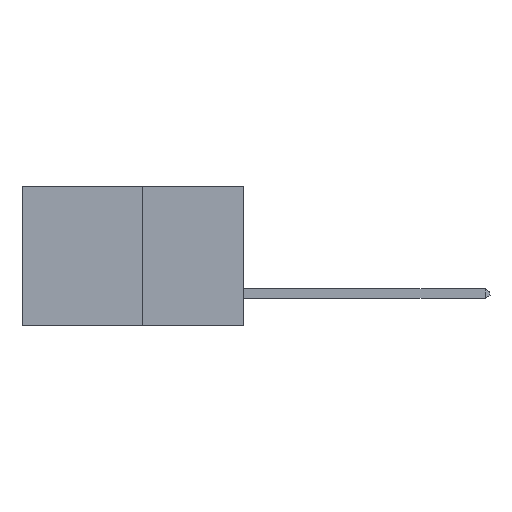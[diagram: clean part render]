
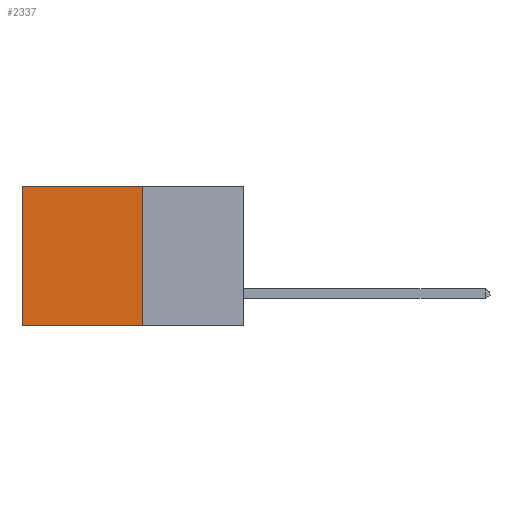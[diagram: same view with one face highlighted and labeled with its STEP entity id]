
A CAD part, left-side view. The second image highlights one B-rep face of the part: STEP entity #2337.
In plain terms, the highlighted planar face has unit normal (-1, 0, 0).
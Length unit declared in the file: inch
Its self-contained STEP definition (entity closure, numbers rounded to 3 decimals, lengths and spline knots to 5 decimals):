
#758 = EDGE_CURVE ( 'NONE', #4293, #9206, #2793, .T. ) ;
#808 = EDGE_LOOP ( 'NONE', ( #9528, #7531, #5480, #3408 ) ) ;
#1374 = CARTESIAN_POINT ( 'NONE',  ( 0.277, 0.27, -0.37 ) ) ;
#1748 = VERTEX_POINT ( 'NONE', #5710 ) ;
#1931 = DIRECTION ( 'NONE',  ( 0., 1., 0. ) ) ;
#2206 = VECTOR ( 'NONE', #9385, 39.37008 ) ;
#2337 = ADVANCED_FACE ( 'NONE', ( #6707 ), #9461, .F. ) ;
#2450 = CARTESIAN_POINT ( 'NONE',  ( 0.277, 0.27, -0.37 ) ) ;
#2793 = LINE ( 'NONE', #1374, #6991 ) ;
#2859 = VERTEX_POINT ( 'NONE', #4908 ) ;
#3236 = CARTESIAN_POINT ( 'NONE',  ( 0.277, 0.27, 0. ) ) ;
#3363 = EDGE_CURVE ( 'NONE', #2859, #9206, #4689, .T. ) ;
#3408 = ORIENTED_EDGE ( 'NONE', *, *, #3448, .T. ) ;
#3444 = LINE ( 'NONE', #3236, #6835 ) ;
#3448 = EDGE_CURVE ( 'NONE', #1748, #2859, #3444, .T. ) ;
#4293 = VERTEX_POINT ( 'NONE', #10232 ) ;
#4609 = DIRECTION ( 'NONE',  ( 0., 1., 0. ) ) ;
#4689 = LINE ( 'NONE', #10209, #2206 ) ;
#4908 = CARTESIAN_POINT ( 'NONE',  ( 0.277, 0.59, 0. ) ) ;
#4949 = DIRECTION ( 'NONE',  ( 0., 0., -1. ) ) ;
#5480 = ORIENTED_EDGE ( 'NONE', *, *, #7205, .F. ) ;
#5710 = CARTESIAN_POINT ( 'NONE',  ( 0.277, 0.27, 0. ) ) ;
#6707 = FACE_OUTER_BOUND ( 'NONE', #808, .T. ) ;
#6835 = VECTOR ( 'NONE', #1931, 39.37008 ) ;
#6991 = VECTOR ( 'NONE', #4609, 39.37008 ) ;
#7042 = CARTESIAN_POINT ( 'NONE',  ( 0.277, 0.27, -0.37 ) ) ;
#7205 = EDGE_CURVE ( 'NONE', #1748, #4293, #7634, .T. ) ;
#7356 = CARTESIAN_POINT ( 'NONE',  ( 0.277, 0.59, -0.37 ) ) ;
#7531 = ORIENTED_EDGE ( 'NONE', *, *, #758, .F. ) ;
#7634 = LINE ( 'NONE', #2450, #9401 ) ;
#9206 = VERTEX_POINT ( 'NONE', #7356 ) ;
#9259 = DIRECTION ( 'NONE',  ( 1., 0., 0. ) ) ;
#9385 = DIRECTION ( 'NONE',  ( 0., 0., -1. ) ) ;
#9401 = VECTOR ( 'NONE', #9495, 39.37008 ) ;
#9461 = PLANE ( 'NONE',  #9525 ) ;
#9495 = DIRECTION ( 'NONE',  ( 0., 0., -1. ) ) ;
#9525 = AXIS2_PLACEMENT_3D ( 'NONE', #7042, #9259, #4949 ) ;
#9528 = ORIENTED_EDGE ( 'NONE', *, *, #3363, .T. ) ;
#10209 = CARTESIAN_POINT ( 'NONE',  ( 0.277, 0.59, -0.37 ) ) ;
#10232 = CARTESIAN_POINT ( 'NONE',  ( 0.277, 0.27, -0.37 ) ) ;
